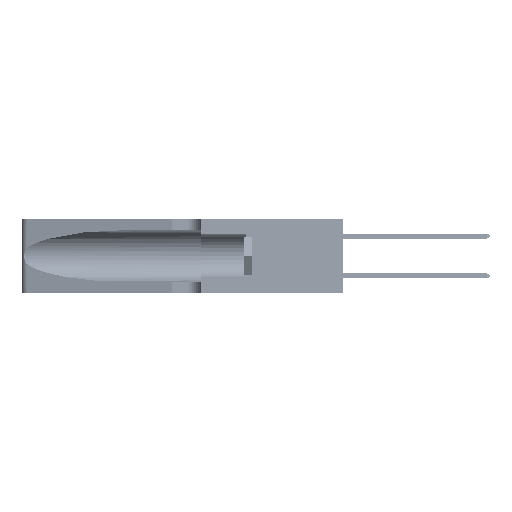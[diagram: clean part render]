
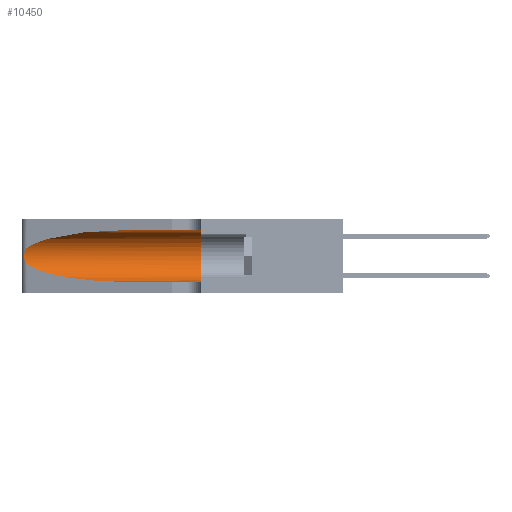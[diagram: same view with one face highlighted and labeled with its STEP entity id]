
A CAD part, left-side view. The second image highlights one B-rep face of the part: STEP entity #10450.
In plain terms, the highlighted cylindrical face has radius 3.308 mm (diameter 6.617 mm), a partial arc.
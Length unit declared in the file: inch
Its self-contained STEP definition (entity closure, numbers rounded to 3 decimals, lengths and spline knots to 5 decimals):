
#203 = CARTESIAN_POINT ( 'NONE',  ( 0.1305, 0.72297, 0.05475 ) ) ;
#1062 = CARTESIAN_POINT ( 'NONE',  ( 0.26075, 1.23896, 0.178 ) ) ;
#1847 = CYLINDRICAL_SURFACE ( 'NONE', #15615, 0.13025 ) ;
#2619 = EDGE_CURVE ( 'NONE', #31828, #24178, #37033, .T. ) ;
#5036 = EDGE_CURVE ( 'NONE', #24178, #29134, #21825, .T. ) ;
#5304 = CARTESIAN_POINT ( 'NONE',  ( 0.25856, 1.23593, 0.16098 ) ) ;
#5916 = CARTESIAN_POINT ( 'NONE',  ( 0.1305, 0.72297, 0.31525 ) ) ;
#7606 = CARTESIAN_POINT ( 'NONE',  ( 0.18966, 0.96281, 0.05475 ) ) ;
#7760 = CARTESIAN_POINT ( 'NONE',  ( 0.1305, 0.35, 0.05475 ) ) ;
#8517 = VECTOR ( 'NONE', #32351, 39.37008 ) ;
#9496 = CARTESIAN_POINT ( 'NONE',  ( 0.25639, 1.23186, 0.15144 ) ) ;
#10071 = EDGE_CURVE ( 'NONE', #29134, #45187, #32426, .T. ) ;
#10450 = ADVANCED_FACE ( 'NONE', ( #34941 ), #1847, .F. ) ;
#11305 = CARTESIAN_POINT ( 'NONE',  ( 0.18966, 0.96281, 0.31525 ) ) ;
#13139 = DIRECTION ( 'NONE',  ( 0., 1., 0. ) ) ;
#13469 = CARTESIAN_POINT ( 'NONE',  ( 0.25487, 1.22718, 0.22369 ) ) ;
#13645 = CARTESIAN_POINT ( 'NONE',  ( 0.25487, 1.22718, 0.14631 ) ) ;
#13791 = CARTESIAN_POINT ( 'NONE',  ( 0.25487, 1.22718, 0.14631 ) ) ;
#14202 = DIRECTION ( 'NONE',  ( 0., 0., -1. ) ) ;
#15615 = AXIS2_PLACEMENT_3D ( 'NONE', #30696, #51267, #14202 ) ;
#17343 = LINE ( 'NONE', #19339, #36660 ) ;
#17498 = ORIENTED_EDGE ( 'NONE', *, *, #40787, .T. ) ;
#17667 = CARTESIAN_POINT ( 'NONE',  ( 0.25639, 1.23184, 0.21858 ) ) ;
#19339 = CARTESIAN_POINT ( 'NONE',  ( 0.1305, 1.61858, 0.31525 ) ) ;
#19789 = EDGE_CURVE ( 'NONE', #30756, #33001, #28834, .T. ) ;
#20631 = ORIENTED_EDGE ( 'NONE', *, *, #19789, .F. ) ;
#21825 = B_SPLINE_CURVE_WITH_KNOTS ( 'NONE', 3,
 ( #13469, #34067, #17667, #46438, #21836, #50556, #26029, #1062, #30160, #5304, #34244, #9496, #38382, #13645 ),
 .UNSPECIFIED., .F., .F.,
 ( 4, 2, 2, 2, 2, 2, 4 ),
 ( 0., 0.00027, 0.00053, 0.00107, 0.0016, 0.00187, 0.00214 ),
 .UNSPECIFIED. ) ;
#21836 = CARTESIAN_POINT ( 'NONE',  ( 0.25854, 1.2359, 0.20912 ) ) ;
#24178 = VERTEX_POINT ( 'NONE', #37697 ) ;
#26029 = CARTESIAN_POINT ( 'NONE',  ( 0.26075, 1.23896, 0.19203 ) ) ;
#28266 = CARTESIAN_POINT ( 'NONE',  ( 0.1305, 1.61858, 0.05475 ) ) ;
#28308 = CARTESIAN_POINT ( 'NONE',  ( 0.25487, 1.22718, 0.14631 ) ) ;
#28419 = EDGE_CURVE ( 'NONE', #31828, #30756, #17343, .T. ) ;
#28834 = CIRCLE ( 'NONE', #35921, 0.13025 ) ;
#29134 = VERTEX_POINT ( 'NONE', #13791 ) ;
#30160 = CARTESIAN_POINT ( 'NONE',  ( 0.26017, 1.23833, 0.17102 ) ) ;
#30547 = ORIENTED_EDGE ( 'NONE', *, *, #10071, .T. ) ;
#30580 = LINE ( 'NONE', #28266, #8517 ) ;
#30696 = CARTESIAN_POINT ( 'NONE',  ( 0.1305, 1.61858, 0.185 ) ) ;
#30756 = VERTEX_POINT ( 'NONE', #52660 ) ;
#31828 = VERTEX_POINT ( 'NONE', #5916 ) ;
#32351 = DIRECTION ( 'NONE',  ( 0., -1., 0. ) ) ;
#32426 =( BOUNDED_CURVE ( )  B_SPLINE_CURVE ( 3, ( #28308, #52807, #7606, #36527 ),
 .UNSPECIFIED., .F., .T. ) 
 B_SPLINE_CURVE_WITH_KNOTS ( ( 4, 4 ),
 ( 3.44316, 4.71239 ),
 .UNSPECIFIED. ) 
 CURVE ( )  GEOMETRIC_REPRESENTATION_ITEM ( )  RATIONAL_B_SPLINE_CURVE ( ( 1., 0.87, 0.87, 1. ) ) 
 REPRESENTATION_ITEM ( '' )  );
#33001 = VERTEX_POINT ( 'NONE', #7760 ) ;
#33236 = EDGE_LOOP ( 'NONE', ( #35050, #53455, #30547, #17498, #20631, #42568 ) ) ;
#34067 = CARTESIAN_POINT ( 'NONE',  ( 0.25555, 1.22994, 0.2215 ) ) ;
#34244 = CARTESIAN_POINT ( 'NONE',  ( 0.25789, 1.23486, 0.15765 ) ) ;
#34941 = FACE_OUTER_BOUND ( 'NONE', #33236, .T. ) ;
#35050 = ORIENTED_EDGE ( 'NONE', *, *, #2619, .T. ) ;
#35921 = AXIS2_PLACEMENT_3D ( 'NONE', #37865, #13139, #41994 ) ;
#36043 = CARTESIAN_POINT ( 'NONE',  ( 0.2373, 1.15595, 0.28018 ) ) ;
#36527 = CARTESIAN_POINT ( 'NONE',  ( 0.1305, 0.72297, 0.05475 ) ) ;
#36660 = VECTOR ( 'NONE', #48105, 39.37008 ) ;
#37033 =( BOUNDED_CURVE ( )  B_SPLINE_CURVE ( 3, ( #39985, #11305, #36043, #40170 ),
 .UNSPECIFIED., .F., .F. ) 
 B_SPLINE_CURVE_WITH_KNOTS ( ( 4, 4 ),
 ( 1.5708, 2.84003 ),
 .UNSPECIFIED. ) 
 CURVE ( )  GEOMETRIC_REPRESENTATION_ITEM ( )  RATIONAL_B_SPLINE_CURVE ( ( 1., 0.87, 0.87, 1. ) ) 
 REPRESENTATION_ITEM ( '' )  );
#37697 = CARTESIAN_POINT ( 'NONE',  ( 0.25487, 1.22718, 0.22369 ) ) ;
#37865 = CARTESIAN_POINT ( 'NONE',  ( 0.1305, 0.35, 0.185 ) ) ;
#38382 = CARTESIAN_POINT ( 'NONE',  ( 0.25555, 1.22993, 0.14849 ) ) ;
#39985 = CARTESIAN_POINT ( 'NONE',  ( 0.1305, 0.72297, 0.31525 ) ) ;
#40170 = CARTESIAN_POINT ( 'NONE',  ( 0.25487, 1.22718, 0.22369 ) ) ;
#40787 = EDGE_CURVE ( 'NONE', #45187, #33001, #30580, .T. ) ;
#41994 = DIRECTION ( 'NONE',  ( 0., 0., 1. ) ) ;
#42568 = ORIENTED_EDGE ( 'NONE', *, *, #28419, .F. ) ;
#45187 = VERTEX_POINT ( 'NONE', #203 ) ;
#46438 = CARTESIAN_POINT ( 'NONE',  ( 0.25787, 1.23484, 0.2124 ) ) ;
#48105 = DIRECTION ( 'NONE',  ( 0., -1., 0. ) ) ;
#50556 = CARTESIAN_POINT ( 'NONE',  ( 0.26018, 1.23835, 0.19895 ) ) ;
#51267 = DIRECTION ( 'NONE',  ( 0., -1., 0. ) ) ;
#52660 = CARTESIAN_POINT ( 'NONE',  ( 0.1305, 0.35, 0.31525 ) ) ;
#52807 = CARTESIAN_POINT ( 'NONE',  ( 0.2373, 1.15595, 0.08982 ) ) ;
#53455 = ORIENTED_EDGE ( 'NONE', *, *, #5036, .T. ) ;
